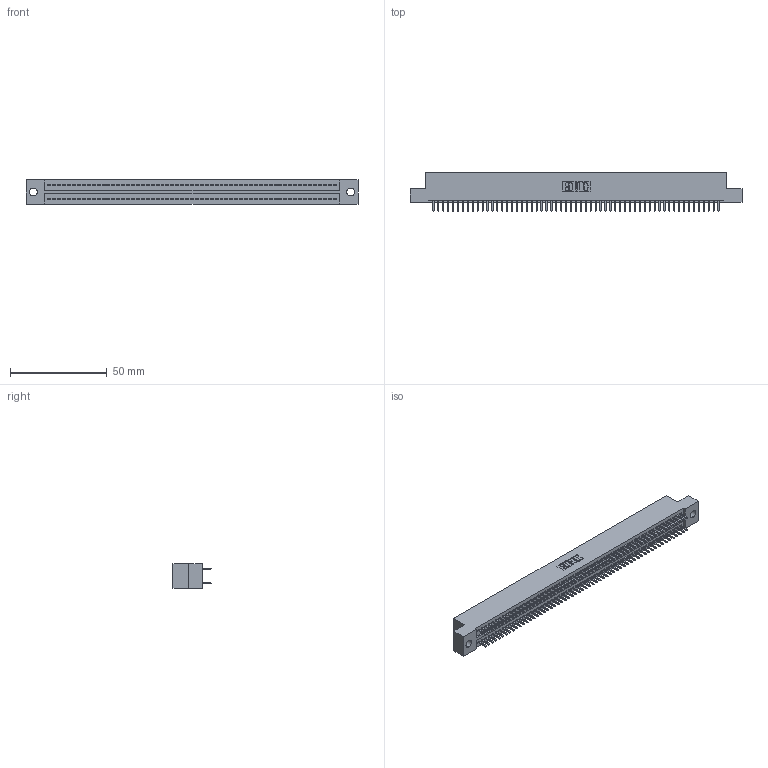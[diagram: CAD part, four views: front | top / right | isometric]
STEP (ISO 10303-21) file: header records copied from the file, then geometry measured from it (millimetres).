
FILE_DESCRIPTION (( 'STEP AP203' ), '1' );
FILE_NAME ('325-118-520-209.STEP', '2020-02-25T08:32:09', ( '' ), ( '' ), 'SwSTEP 2.0', 'SolidWorks 2016', '' );
FILE_SCHEMA (( 'CONFIG_CONTROL_DESIGN' ));
Length unit declared in the file: inch
Products named in the file (3): 325-292-001_325-293-120; 325 Part_.160 TH; 325-118-520-209
Assembly tree (119 placements, depth 2):
  325-118-520-209
    325 Part_.160 TH
    325-292-001_325-293-120  x118
Bounding box: 171.58 x 19.68 x 12.45 mm (x, y, z)
Volume: 22053.9 mm3; surface area: 26778.4 mm2
Topology: 119 solids, 119 shells, 6250 faces, 18601 edges, 12242 vertices
Faces by surface type: plane 4318, cylinder 1932
Entity records: 35779 total; most frequent: CARTESIAN_POINT 5910, ORIENTED_EDGE 5846, DIRECTION 5019, EDGE_CURVE 2923, LINE 2795, VECTOR 2795, VERTEX_POINT 1946, AXIS2_PLACEMENT_3D 1112
